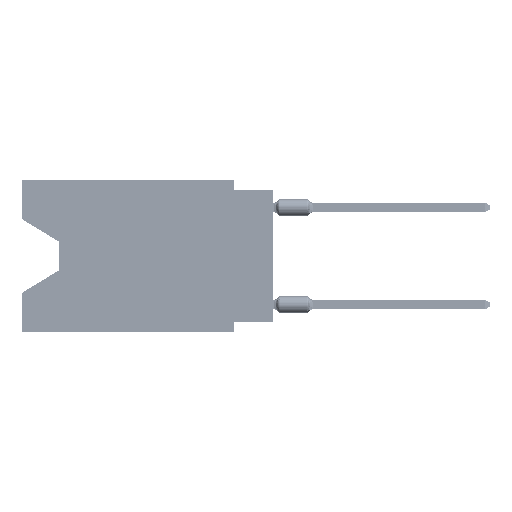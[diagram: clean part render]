
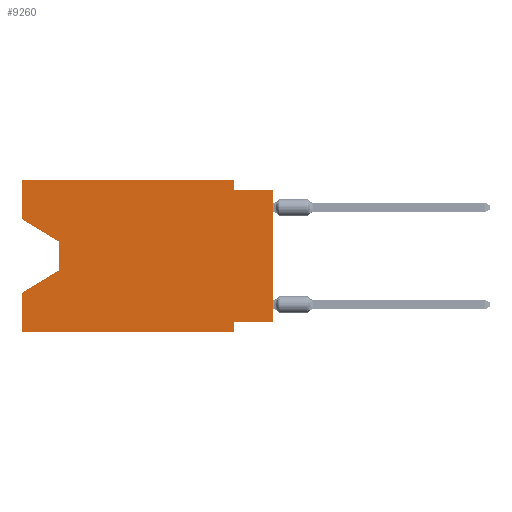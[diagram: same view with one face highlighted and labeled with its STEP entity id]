
A CAD part, left-side view. The second image highlights one B-rep face of the part: STEP entity #9260.
In plain terms, the highlighted planar face has unit normal (-1, 0, 0).
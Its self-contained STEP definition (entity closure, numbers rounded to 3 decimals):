
#71 = CARTESIAN_POINT ( 'NONE',  ( 0., 16.383, -9.906 ) ) ;
#139 = PLANE ( 'NONE',  #69304 ) ;
#152 = CARTESIAN_POINT ( 'NONE',  ( 0., 16.383, 0. ) ) ;
#1416 = DIRECTION ( 'NONE',  ( 1., 0., 0. ) ) ;
#2417 = ORIENTED_EDGE ( 'NONE', *, *, #51394, .F. ) ;
#2768 = CARTESIAN_POINT ( 'NONE',  ( 0., 16.383, -2.546 ) ) ;
#4177 = DIRECTION ( 'NONE',  ( 0., 0., 1. ) ) ;
#6838 = CARTESIAN_POINT ( 'NONE',  ( 0., 0., -0.635 ) ) ;
#7608 = VECTOR ( 'NONE', #73741, 1000. ) ;
#8473 = CARTESIAN_POINT ( 'NONE',  ( 0., 2.54, -9.906 ) ) ;
#8707 = CARTESIAN_POINT ( 'NONE',  ( 0., 16.383, -2.546 ) ) ;
#9260 = ADVANCED_FACE ( 'NONE', ( #58673 ), #139, .F. ) ;
#11668 = VERTEX_POINT ( 'NONE', #21130 ) ;
#12077 = VECTOR ( 'NONE', #52072, 1000. ) ;
#12294 = VECTOR ( 'NONE', #33502, 1000. ) ;
#12561 = LINE ( 'NONE', #152, #22326 ) ;
#13350 = VERTEX_POINT ( 'NONE', #20766 ) ;
#14142 = ORIENTED_EDGE ( 'NONE', *, *, #73370, .F. ) ;
#14874 = LINE ( 'NONE', #48135, #34657 ) ;
#14944 = DIRECTION ( 'NONE',  ( 0., -1., 0. ) ) ;
#15577 = VECTOR ( 'NONE', #22388, 1000. ) ;
#19277 = CARTESIAN_POINT ( 'NONE',  ( 0., 13.97, -5.893 ) ) ;
#19330 = ORIENTED_EDGE ( 'NONE', *, *, #22363, .F. ) ;
#19453 = VERTEX_POINT ( 'NONE', #19804 ) ;
#19804 = CARTESIAN_POINT ( 'NONE',  ( 0., 0., -9.271 ) ) ;
#20766 = CARTESIAN_POINT ( 'NONE',  ( 0., 16.383, -7.36 ) ) ;
#20849 = EDGE_CURVE ( 'NONE', #55699, #23190, #14874, .T. ) ;
#21130 = CARTESIAN_POINT ( 'NONE',  ( 0., 2.54, 0. ) ) ;
#21741 = EDGE_CURVE ( 'NONE', #19453, #29031, #57599, .T. ) ;
#22326 = VECTOR ( 'NONE', #39861, 1000. ) ;
#22363 = EDGE_CURVE ( 'NONE', #19453, #73251, #47662, .T. ) ;
#22388 = DIRECTION ( 'NONE',  ( 0., 0., -1. ) ) ;
#23190 = VERTEX_POINT ( 'NONE', #19277 ) ;
#23237 = ORIENTED_EDGE ( 'NONE', *, *, #75400, .F. ) ;
#25125 = CARTESIAN_POINT ( 'NONE',  ( 0., 0., 0. ) ) ;
#26190 = DIRECTION ( 'NONE',  ( 0., 0., -1. ) ) ;
#26337 = ORIENTED_EDGE ( 'NONE', *, *, #68002, .T. ) ;
#27081 = ORIENTED_EDGE ( 'NONE', *, *, #34489, .F. ) ;
#27690 = CARTESIAN_POINT ( 'NONE',  ( 0., 2.54, -9.271 ) ) ;
#28571 = CARTESIAN_POINT ( 'NONE',  ( 0., 13.97, -5.893 ) ) ;
#28812 = LINE ( 'NONE', #80934, #15577 ) ;
#29031 = VERTEX_POINT ( 'NONE', #45389 ) ;
#30842 = LINE ( 'NONE', #71, #84473 ) ;
#33502 = DIRECTION ( 'NONE',  ( 0., -0.855, -0.519 ) ) ;
#34476 = VERTEX_POINT ( 'NONE', #2768 ) ;
#34489 = EDGE_CURVE ( 'NONE', #11668, #35775, #28812, .T. ) ;
#34657 = VECTOR ( 'NONE', #74217, 1000. ) ;
#35775 = VERTEX_POINT ( 'NONE', #42112 ) ;
#37240 = DIRECTION ( 'NONE',  ( 0., -1., 0. ) ) ;
#37531 = VECTOR ( 'NONE', #14944, 1000. ) ;
#39861 = DIRECTION ( 'NONE',  ( 0., 0., 1. ) ) ;
#40528 = VERTEX_POINT ( 'NONE', #64094 ) ;
#42112 = CARTESIAN_POINT ( 'NONE',  ( 0., 2.54, -0.635 ) ) ;
#43469 = VECTOR ( 'NONE', #4177, 1000. ) ;
#45389 = CARTESIAN_POINT ( 'NONE',  ( 0., 0., -0.635 ) ) ;
#46936 = DIRECTION ( 'NONE',  ( 0., 0.855, -0.519 ) ) ;
#47662 = LINE ( 'NONE', #54065, #7608 ) ;
#48003 = LINE ( 'NONE', #8707, #12294 ) ;
#48135 = CARTESIAN_POINT ( 'NONE',  ( 0., 13.97, -4.013 ) ) ;
#49554 = DIRECTION ( 'NONE',  ( 0., 0., -1. ) ) ;
#50391 = CARTESIAN_POINT ( 'NONE',  ( 0., 13.97, -4.013 ) ) ;
#50554 = VECTOR ( 'NONE', #49554, 1000. ) ;
#51193 = DIRECTION ( 'NONE',  ( 0., 0., 1. ) ) ;
#51394 = EDGE_CURVE ( 'NONE', #35775, #29031, #65361, .T. ) ;
#51676 = ORIENTED_EDGE ( 'NONE', *, *, #21741, .T. ) ;
#52072 = DIRECTION ( 'NONE',  ( 0., -1., 0. ) ) ;
#52315 = VERTEX_POINT ( 'NONE', #8473 ) ;
#52486 = LINE ( 'NONE', #71719, #12077 ) ;
#54065 = CARTESIAN_POINT ( 'NONE',  ( 0., 0., -9.271 ) ) ;
#54612 = LINE ( 'NONE', #69531, #43469 ) ;
#55699 = VERTEX_POINT ( 'NONE', #50391 ) ;
#57599 = LINE ( 'NONE', #25125, #68877 ) ;
#58673 = FACE_OUTER_BOUND ( 'NONE', #69452, .T. ) ;
#60964 = EDGE_CURVE ( 'NONE', #34476, #55699, #48003, .T. ) ;
#63014 = ORIENTED_EDGE ( 'NONE', *, *, #73227, .F. ) ;
#63592 = ORIENTED_EDGE ( 'NONE', *, *, #20849, .T. ) ;
#64094 = CARTESIAN_POINT ( 'NONE',  ( 0., 16.383, 0. ) ) ;
#65221 = VERTEX_POINT ( 'NONE', #81965 ) ;
#65361 = LINE ( 'NONE', #6838, #37531 ) ;
#68002 = EDGE_CURVE ( 'NONE', #65221, #52315, #30842, .T. ) ;
#68302 = VECTOR ( 'NONE', #46936, 1000. ) ;
#68877 = VECTOR ( 'NONE', #51193, 1000. ) ;
#69304 = AXIS2_PLACEMENT_3D ( 'NONE', #71911, #1416, #26190 ) ;
#69452 = EDGE_LOOP ( 'NONE', ( #83950, #63592, #76586, #14142, #26337, #23237, #19330, #51676, #2417, #27081, #63014, #78886 ) ) ;
#69531 = CARTESIAN_POINT ( 'NONE',  ( 0., 16.383, 0. ) ) ;
#71719 = CARTESIAN_POINT ( 'NONE',  ( 0., 16.383, 0. ) ) ;
#71911 = CARTESIAN_POINT ( 'NONE',  ( 0., 16.383, 0. ) ) ;
#73227 = EDGE_CURVE ( 'NONE', #40528, #11668, #52486, .T. ) ;
#73251 = VERTEX_POINT ( 'NONE', #27690 ) ;
#73370 = EDGE_CURVE ( 'NONE', #65221, #13350, #54612, .T. ) ;
#73741 = DIRECTION ( 'NONE',  ( 0., 1., 0. ) ) ;
#74217 = DIRECTION ( 'NONE',  ( 0., 0., -1. ) ) ;
#75400 = EDGE_CURVE ( 'NONE', #73251, #52315, #82900, .T. ) ;
#75592 = EDGE_CURVE ( 'NONE', #23190, #13350, #79843, .T. ) ;
#76586 = ORIENTED_EDGE ( 'NONE', *, *, #75592, .T. ) ;
#78886 = ORIENTED_EDGE ( 'NONE', *, *, #84277, .F. ) ;
#79843 = LINE ( 'NONE', #28571, #68302 ) ;
#80934 = CARTESIAN_POINT ( 'NONE',  ( 0., 2.54, 0. ) ) ;
#81965 = CARTESIAN_POINT ( 'NONE',  ( 0., 16.383, -9.906 ) ) ;
#82055 = CARTESIAN_POINT ( 'NONE',  ( 0., 2.54, -9.906 ) ) ;
#82900 = LINE ( 'NONE', #82055, #50554 ) ;
#83950 = ORIENTED_EDGE ( 'NONE', *, *, #60964, .T. ) ;
#84277 = EDGE_CURVE ( 'NONE', #34476, #40528, #12561, .T. ) ;
#84473 = VECTOR ( 'NONE', #37240, 1000. ) ;
